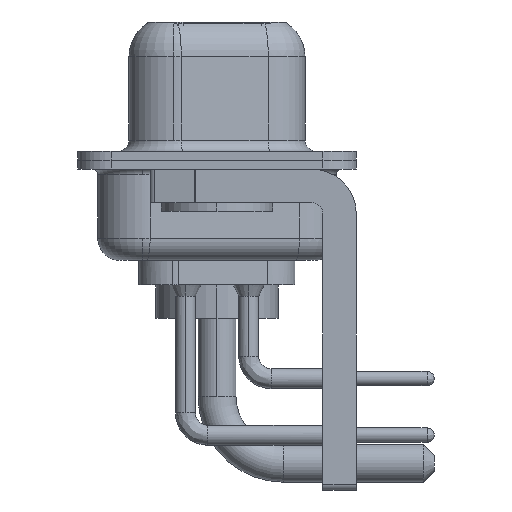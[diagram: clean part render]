
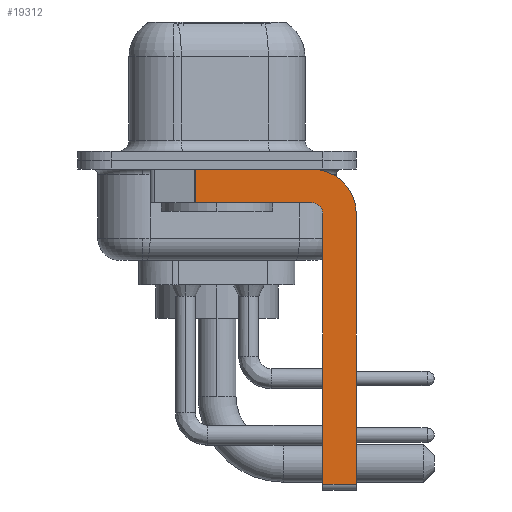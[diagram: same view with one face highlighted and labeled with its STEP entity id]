
A CAD part, left-side view. The second image highlights one B-rep face of the part: STEP entity #19312.
In plain terms, the highlighted planar face has unit normal (-1, 0, 0).
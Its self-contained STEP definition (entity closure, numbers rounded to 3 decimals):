
#14 = CARTESIAN_POINT ( 'NONE',  ( -2.9, -4.25, -2.4 ) ) ;
#312 = CIRCLE ( 'NONE', #623, 0.5 ) ;
#623 = AXIS2_PLACEMENT_3D ( 'NONE', #17798, #19170, #11731 ) ;
#675 = EDGE_CURVE ( 'NONE', #16941, #11699, #10883, .T. ) ;
#1682 = CIRCLE ( 'NONE', #2310, 2. ) ;
#1740 = CARTESIAN_POINT ( 'NONE',  ( -2.9, 0.978, -0.4 ) ) ;
#2136 = VECTOR ( 'NONE', #3301, 1000. ) ;
#2229 = EDGE_CURVE ( 'NONE', #13282, #10332, #8479, .T. ) ;
#2310 = AXIS2_PLACEMENT_3D ( 'NONE', #14, #13798, #3168 ) ;
#2765 = VERTEX_POINT ( 'NONE', #1740 ) ;
#3168 = DIRECTION ( 'NONE',  ( 0., 0., -1. ) ) ;
#3301 = DIRECTION ( 'NONE',  ( 0., -1., 0. ) ) ;
#3306 = VECTOR ( 'NONE', #7467, 1000. ) ;
#3389 = EDGE_CURVE ( 'NONE', #13282, #8601, #6428, .T. ) ;
#4156 = ORIENTED_EDGE ( 'NONE', *, *, #15191, .F. ) ;
#4389 = ORIENTED_EDGE ( 'NONE', *, *, #9311, .F. ) ;
#4499 = VERTEX_POINT ( 'NONE', #15733 ) ;
#4772 = CARTESIAN_POINT ( 'NONE',  ( -2.9, -4.25, -1.9 ) ) ;
#5322 = CARTESIAN_POINT ( 'NONE',  ( -2.9, -4.75, -2.4 ) ) ;
#5367 = VECTOR ( 'NONE', #10700, 1000. ) ;
#5591 = EDGE_CURVE ( 'NONE', #9722, #4499, #1682, .T. ) ;
#5996 = DIRECTION ( 'NONE',  ( 0., -1., 0. ) ) ;
#6042 = CARTESIAN_POINT ( 'NONE',  ( -2.9, -4.25, -0.4 ) ) ;
#6428 = LINE ( 'NONE', #18255, #2136 ) ;
#7204 = EDGE_CURVE ( 'NONE', #2765, #11699, #18201, .T. ) ;
#7467 = DIRECTION ( 'NONE',  ( 0., 0., -1. ) ) ;
#8135 = ORIENTED_EDGE ( 'NONE', *, *, #5591, .F. ) ;
#8479 = LINE ( 'NONE', #16235, #16488 ) ;
#8601 = VERTEX_POINT ( 'NONE', #12339 ) ;
#9311 = EDGE_CURVE ( 'NONE', #2765, #9722, #16509, .T. ) ;
#9722 = VERTEX_POINT ( 'NONE', #6042 ) ;
#10065 = ORIENTED_EDGE ( 'NONE', *, *, #3389, .T. ) ;
#10067 = CARTESIAN_POINT ( 'NONE',  ( -2.9, -4.75, -14.55 ) ) ;
#10332 = VERTEX_POINT ( 'NONE', #5322 ) ;
#10387 = FACE_OUTER_BOUND ( 'NONE', #13804, .T. ) ;
#10516 = ORIENTED_EDGE ( 'NONE', *, *, #7204, .T. ) ;
#10700 = DIRECTION ( 'NONE',  ( 0., 0., -1. ) ) ;
#10883 = LINE ( 'NONE', #4772, #15598 ) ;
#11439 = AXIS2_PLACEMENT_3D ( 'NONE', #17857, #17656, #13351 ) ;
#11551 = DIRECTION ( 'NONE',  ( 0., 0., 1. ) ) ;
#11699 = VERTEX_POINT ( 'NONE', #17517 ) ;
#11731 = DIRECTION ( 'NONE',  ( 0., 0., 1. ) ) ;
#11782 = PLANE ( 'NONE',  #11439 ) ;
#12339 = CARTESIAN_POINT ( 'NONE',  ( -2.9, -6.25, -14.55 ) ) ;
#12452 = ORIENTED_EDGE ( 'NONE', *, *, #2229, .F. ) ;
#13282 = VERTEX_POINT ( 'NONE', #10067 ) ;
#13351 = DIRECTION ( 'NONE',  ( 0., 0., -1. ) ) ;
#13398 = CARTESIAN_POINT ( 'NONE',  ( -2.9, 0.978, -1.9 ) ) ;
#13798 = DIRECTION ( 'NONE',  ( 1., 0., 0. ) ) ;
#13804 = EDGE_LOOP ( 'NONE', ( #4389, #10516, #15721, #4156, #12452, #10065, #16717, #8135 ) ) ;
#13837 = DIRECTION ( 'NONE',  ( 0., 1., 0. ) ) ;
#13941 = LINE ( 'NONE', #18172, #5367 ) ;
#15191 = EDGE_CURVE ( 'NONE', #10332, #16941, #312, .T. ) ;
#15248 = CARTESIAN_POINT ( 'NONE',  ( -2.9, 3., -0.4 ) ) ;
#15598 = VECTOR ( 'NONE', #13837, 1000. ) ;
#15721 = ORIENTED_EDGE ( 'NONE', *, *, #675, .F. ) ;
#15733 = CARTESIAN_POINT ( 'NONE',  ( -2.9, -6.25, -2.4 ) ) ;
#15821 = EDGE_CURVE ( 'NONE', #4499, #8601, #13941, .T. ) ;
#16235 = CARTESIAN_POINT ( 'NONE',  ( -2.9, -4.75, -14.8 ) ) ;
#16488 = VECTOR ( 'NONE', #11551, 1000. ) ;
#16509 = LINE ( 'NONE', #15248, #19082 ) ;
#16717 = ORIENTED_EDGE ( 'NONE', *, *, #15821, .F. ) ;
#16941 = VERTEX_POINT ( 'NONE', #18479 ) ;
#17517 = CARTESIAN_POINT ( 'NONE',  ( -2.9, 0.978, -1.9 ) ) ;
#17656 = DIRECTION ( 'NONE',  ( 1., 0., 0. ) ) ;
#17798 = CARTESIAN_POINT ( 'NONE',  ( -2.9, -4.25, -2.4 ) ) ;
#17857 = CARTESIAN_POINT ( 'NONE',  ( -2.9, -4.25, -2.4 ) ) ;
#18172 = CARTESIAN_POINT ( 'NONE',  ( -2.9, -6.25, -2.4 ) ) ;
#18201 = LINE ( 'NONE', #13398, #3306 ) ;
#18255 = CARTESIAN_POINT ( 'NONE',  ( -2.9, -4.25, -14.55 ) ) ;
#18479 = CARTESIAN_POINT ( 'NONE',  ( -2.9, -4.25, -1.9 ) ) ;
#19082 = VECTOR ( 'NONE', #5996, 1000. ) ;
#19170 = DIRECTION ( 'NONE',  ( -1., 0., 0. ) ) ;
#19312 = ADVANCED_FACE ( 'NONE', ( #10387 ), #11782, .F. ) ;
